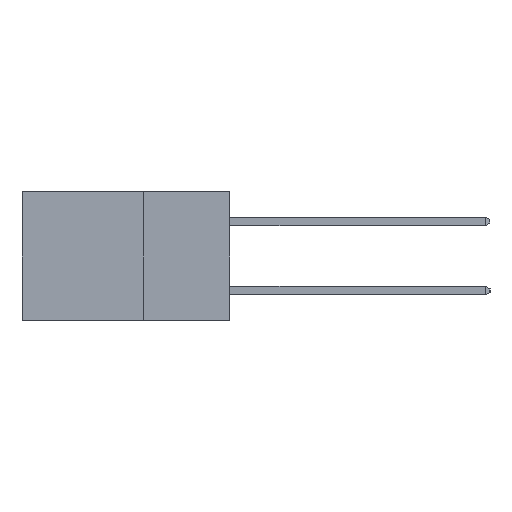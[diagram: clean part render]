
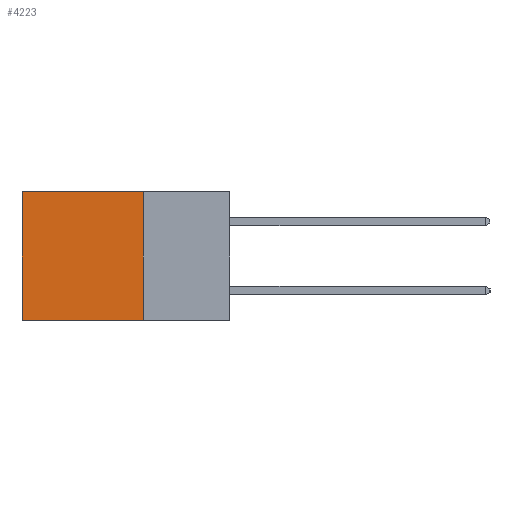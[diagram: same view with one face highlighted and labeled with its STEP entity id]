
A CAD part, left-side view. The second image highlights one B-rep face of the part: STEP entity #4223.
In plain terms, the highlighted planar face has unit normal (-1, 0, 0).
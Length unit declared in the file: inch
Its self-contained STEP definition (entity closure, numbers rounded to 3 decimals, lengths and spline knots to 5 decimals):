
#469 = FACE_OUTER_BOUND ( 'NONE', #2137, .T. ) ;
#809 = ORIENTED_EDGE ( 'NONE', *, *, #5873, .T. ) ;
#1213 = VECTOR ( 'NONE', #12794, 39.37008 ) ;
#1308 = EDGE_CURVE ( 'NONE', #8766, #3209, #14211, .T. ) ;
#1322 = LINE ( 'NONE', #11939, #4895 ) ;
#1728 = ORIENTED_EDGE ( 'NONE', *, *, #1308, .F. ) ;
#1898 = ORIENTED_EDGE ( 'NONE', *, *, #4203, .T. ) ;
#2137 = EDGE_LOOP ( 'NONE', ( #1898, #15360, #1728, #809 ) ) ;
#2488 = CARTESIAN_POINT ( 'NONE',  ( 0.2615, 0.25, -0.37 ) ) ;
#3209 = VERTEX_POINT ( 'NONE', #16290 ) ;
#3395 = VECTOR ( 'NONE', #4856, 39.37008 ) ;
#4203 = EDGE_CURVE ( 'NONE', #11687, #12915, #1322, .T. ) ;
#4223 = ADVANCED_FACE ( 'NONE', ( #469 ), #11744, .F. ) ;
#4772 = CARTESIAN_POINT ( 'NONE',  ( 0.2615, 0.25, 0. ) ) ;
#4856 = DIRECTION ( 'NONE',  ( 0., 1., 0. ) ) ;
#4895 = VECTOR ( 'NONE', #11838, 39.37008 ) ;
#5873 = EDGE_CURVE ( 'NONE', #8766, #11687, #6853, .T. ) ;
#6853 = LINE ( 'NONE', #4772, #3395 ) ;
#7028 = CARTESIAN_POINT ( 'NONE',  ( 0.2615, 0.25, 0. ) ) ;
#7512 = VECTOR ( 'NONE', #12800, 39.37008 ) ;
#8766 = VERTEX_POINT ( 'NONE', #7028 ) ;
#10146 = CARTESIAN_POINT ( 'NONE',  ( 0.2615, 0.6, 0. ) ) ;
#11426 = CARTESIAN_POINT ( 'NONE',  ( 0.2615, 0.6, -0.37 ) ) ;
#11630 = DIRECTION ( 'NONE',  ( 0., 0., -1. ) ) ;
#11666 = DIRECTION ( 'NONE',  ( 1., 0., 0. ) ) ;
#11687 = VERTEX_POINT ( 'NONE', #10146 ) ;
#11719 = CARTESIAN_POINT ( 'NONE',  ( 0.2615, 0.25, -0.37 ) ) ;
#11744 = PLANE ( 'NONE',  #12615 ) ;
#11838 = DIRECTION ( 'NONE',  ( 0., 0., -1. ) ) ;
#11939 = CARTESIAN_POINT ( 'NONE',  ( 0.2615, 0.6, -0.37 ) ) ;
#12615 = AXIS2_PLACEMENT_3D ( 'NONE', #11719, #11666, #11630 ) ;
#12794 = DIRECTION ( 'NONE',  ( 0., 1., 0. ) ) ;
#12800 = DIRECTION ( 'NONE',  ( 0., 0., -1. ) ) ;
#12915 = VERTEX_POINT ( 'NONE', #11426 ) ;
#14211 = LINE ( 'NONE', #15658, #7512 ) ;
#14862 = LINE ( 'NONE', #2488, #1213 ) ;
#15348 = EDGE_CURVE ( 'NONE', #3209, #12915, #14862, .T. ) ;
#15360 = ORIENTED_EDGE ( 'NONE', *, *, #15348, .F. ) ;
#15658 = CARTESIAN_POINT ( 'NONE',  ( 0.2615, 0.25, -0.37 ) ) ;
#16290 = CARTESIAN_POINT ( 'NONE',  ( 0.2615, 0.25, -0.37 ) ) ;
